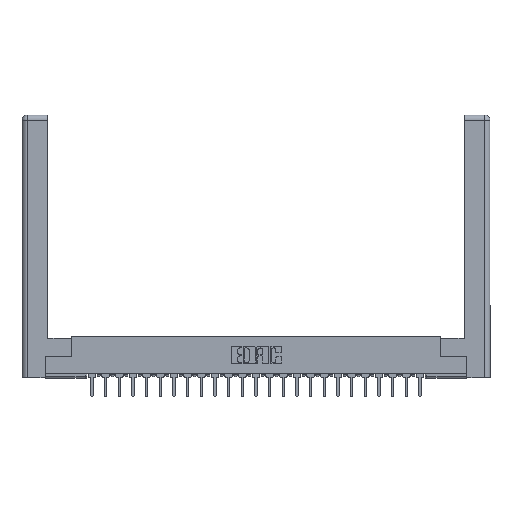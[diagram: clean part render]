
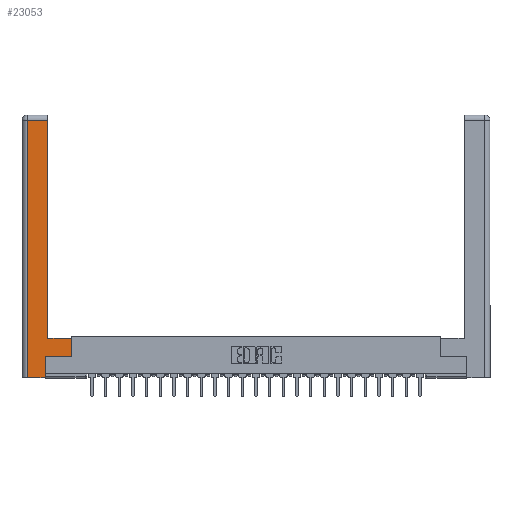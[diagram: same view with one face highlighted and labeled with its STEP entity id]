
A CAD part, top view. The second image highlights one B-rep face of the part: STEP entity #23053.
In plain terms, the highlighted planar face has unit normal (0, 0, 1).
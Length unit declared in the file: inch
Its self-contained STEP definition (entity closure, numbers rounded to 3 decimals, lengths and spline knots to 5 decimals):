
#101 = ORIENTED_EDGE ( 'NONE', *, *, #18146, .T. ) ;
#420 = CARTESIAN_POINT ( 'NONE',  ( 0.0615, 0., 0. ) ) ;
#478 = CARTESIAN_POINT ( 'NONE',  ( 0.565, 0.245, 0. ) ) ;
#773 = CARTESIAN_POINT ( 'NONE',  ( 0.0615, 2.94, 0. ) ) ;
#776 = CARTESIAN_POINT ( 'NONE',  ( 0.0615, 2.94, 0. ) ) ;
#1560 = VECTOR ( 'NONE', #26877, 39.37008 ) ;
#2741 = CARTESIAN_POINT ( 'NONE',  ( 0.0615, 0., 0. ) ) ;
#3614 = VERTEX_POINT ( 'NONE', #10203 ) ;
#4529 = CARTESIAN_POINT ( 'NONE',  ( 0.295, 0.45, 0. ) ) ;
#5281 = VERTEX_POINT ( 'NONE', #773 ) ;
#5433 = EDGE_CURVE ( 'NONE', #3614, #5281, #8487, .T. ) ;
#5552 = LINE ( 'NONE', #9888, #19528 ) ;
#6074 = DIRECTION ( 'NONE',  ( 0., 0., -1. ) ) ;
#6234 = VERTEX_POINT ( 'NONE', #25080 ) ;
#6262 = EDGE_CURVE ( 'NONE', #14720, #3614, #22436, .T. ) ;
#6344 = EDGE_CURVE ( 'NONE', #8656, #18325, #17533, .T. ) ;
#7990 = CARTESIAN_POINT ( 'NONE',  ( 0., 0., 0. ) ) ;
#8155 = DIRECTION ( 'NONE',  ( 1., 0., 0. ) ) ;
#8196 = EDGE_LOOP ( 'NONE', ( #20904, #10921, #20828, #20192, #12210, #101, #15434, #13301 ) ) ;
#8265 = PLANE ( 'NONE',  #18085 ) ;
#8487 = LINE ( 'NONE', #776, #18547 ) ;
#8656 = VERTEX_POINT ( 'NONE', #420 ) ;
#8715 = CARTESIAN_POINT ( 'NONE',  ( 0.565, 0.45, 0. ) ) ;
#9888 = CARTESIAN_POINT ( 'NONE',  ( 0.565, 0.245, 0. ) ) ;
#10203 = CARTESIAN_POINT ( 'NONE',  ( 0.295, 2.94, 0. ) ) ;
#10588 = DIRECTION ( 'NONE',  ( 1., 0., 0. ) ) ;
#10762 = DIRECTION ( 'NONE',  ( 0., 1., 0. ) ) ;
#10921 = ORIENTED_EDGE ( 'NONE', *, *, #5433, .T. ) ;
#11198 = VECTOR ( 'NONE', #25687, 39.37008 ) ;
#12188 = LINE ( 'NONE', #23859, #11198 ) ;
#12210 = ORIENTED_EDGE ( 'NONE', *, *, #13432, .T. ) ;
#12320 = CARTESIAN_POINT ( 'NONE',  ( 0.295, 3., 0. ) ) ;
#12554 = FACE_OUTER_BOUND ( 'NONE', #8196, .T. ) ;
#12789 = CARTESIAN_POINT ( 'NONE',  ( 0.265, 0., 0. ) ) ;
#13301 = ORIENTED_EDGE ( 'NONE', *, *, #14254, .T. ) ;
#13432 = EDGE_CURVE ( 'NONE', #18325, #6234, #20997, .T. ) ;
#14254 = EDGE_CURVE ( 'NONE', #24590, #14720, #12188, .T. ) ;
#14720 = VERTEX_POINT ( 'NONE', #4529 ) ;
#14847 = LINE ( 'NONE', #23055, #23027 ) ;
#15343 = DIRECTION ( 'NONE',  ( -1., 0., 0. ) ) ;
#15434 = ORIENTED_EDGE ( 'NONE', *, *, #22545, .T. ) ;
#15796 = VERTEX_POINT ( 'NONE', #478 ) ;
#17036 = CARTESIAN_POINT ( 'NONE',  ( 0.265, 0.245, 0. ) ) ;
#17533 = LINE ( 'NONE', #25167, #26334 ) ;
#18085 = AXIS2_PLACEMENT_3D ( 'NONE', #7990, #6074, #22844 ) ;
#18146 = EDGE_CURVE ( 'NONE', #6234, #15796, #5552, .T. ) ;
#18164 = VECTOR ( 'NONE', #25787, 39.37008 ) ;
#18325 = VERTEX_POINT ( 'NONE', #12789 ) ;
#18547 = VECTOR ( 'NONE', #15343, 39.37008 ) ;
#19125 = EDGE_CURVE ( 'NONE', #5281, #8656, #23750, .T. ) ;
#19528 = VECTOR ( 'NONE', #8155, 39.37008 ) ;
#19664 = VECTOR ( 'NONE', #10762, 39.37008 ) ;
#20192 = ORIENTED_EDGE ( 'NONE', *, *, #6344, .T. ) ;
#20828 = ORIENTED_EDGE ( 'NONE', *, *, #19125, .T. ) ;
#20904 = ORIENTED_EDGE ( 'NONE', *, *, #6262, .T. ) ;
#20997 = LINE ( 'NONE', #17036, #19664 ) ;
#22436 = LINE ( 'NONE', #12320, #1560 ) ;
#22545 = EDGE_CURVE ( 'NONE', #15796, #24590, #14847, .T. ) ;
#22844 = DIRECTION ( 'NONE',  ( -1., 0., 0. ) ) ;
#23027 = VECTOR ( 'NONE', #25141, 39.37008 ) ;
#23053 = ADVANCED_FACE ( 'NONE', ( #12554 ), #8265, .F. ) ;
#23055 = CARTESIAN_POINT ( 'NONE',  ( 0.565, 0.45, 0. ) ) ;
#23750 = LINE ( 'NONE', #2741, #18164 ) ;
#23859 = CARTESIAN_POINT ( 'NONE',  ( 0.295, 0.45, 0. ) ) ;
#24590 = VERTEX_POINT ( 'NONE', #8715 ) ;
#25080 = CARTESIAN_POINT ( 'NONE',  ( 0.265, 0.245, 0. ) ) ;
#25141 = DIRECTION ( 'NONE',  ( 0., 1., 0. ) ) ;
#25167 = CARTESIAN_POINT ( 'NONE',  ( 0.265, 0., 0. ) ) ;
#25687 = DIRECTION ( 'NONE',  ( -1., 0., 0. ) ) ;
#25787 = DIRECTION ( 'NONE',  ( 0., -1., 0. ) ) ;
#26334 = VECTOR ( 'NONE', #10588, 39.37008 ) ;
#26877 = DIRECTION ( 'NONE',  ( 0., 1., 0. ) ) ;
